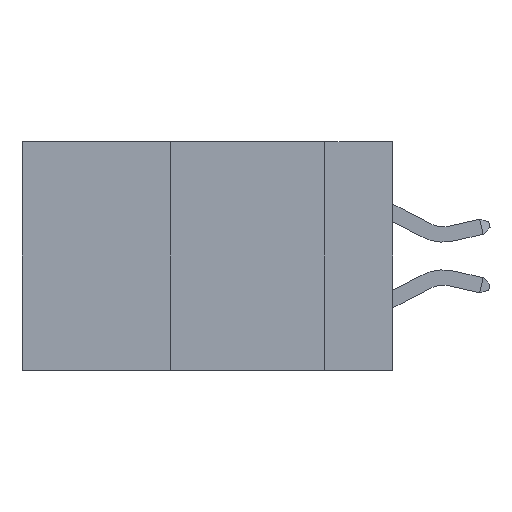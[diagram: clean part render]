
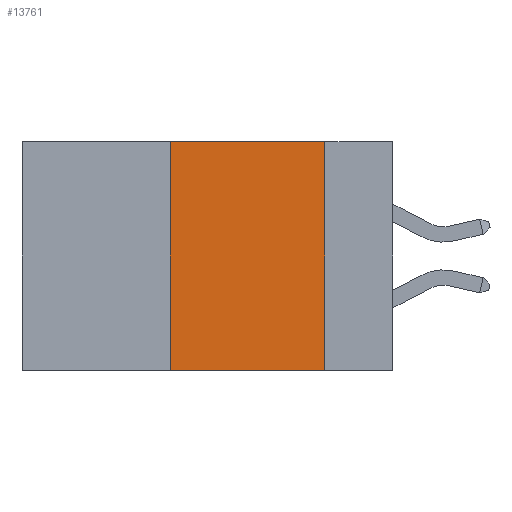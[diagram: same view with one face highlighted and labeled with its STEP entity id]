
A CAD part, left-side view. The second image highlights one B-rep face of the part: STEP entity #13761.
In plain terms, the highlighted planar face has unit normal (-1, 0, 0).
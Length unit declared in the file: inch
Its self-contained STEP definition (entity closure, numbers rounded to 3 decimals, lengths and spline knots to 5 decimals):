
#964 = DIRECTION ( 'NONE',  ( 1., 0., 0. ) ) ;
#1070 = VECTOR ( 'NONE', #2989, 39.37008 ) ;
#1494 = ORIENTED_EDGE ( 'NONE', *, *, #7366, .F. ) ;
#1691 = LINE ( 'NONE', #11585, #4032 ) ;
#1706 = CARTESIAN_POINT ( 'NONE',  ( 0., 0.36, 0. ) ) ;
#2989 = DIRECTION ( 'NONE',  ( 0., 0., 1. ) ) ;
#4032 = VECTOR ( 'NONE', #7355, 39.37008 ) ;
#4509 = ORIENTED_EDGE ( 'NONE', *, *, #10254, .T. ) ;
#5245 = CARTESIAN_POINT ( 'NONE',  ( 0., 0.11, -0.37 ) ) ;
#5344 = VERTEX_POINT ( 'NONE', #13307 ) ;
#5580 = CARTESIAN_POINT ( 'NONE',  ( 0., 0.36, 0. ) ) ;
#5608 = VECTOR ( 'NONE', #14240, 39.37008 ) ;
#6474 = ORIENTED_EDGE ( 'NONE', *, *, #16320, .F. ) ;
#7355 = DIRECTION ( 'NONE',  ( 0., -1., 0. ) ) ;
#7366 = EDGE_CURVE ( 'NONE', #11737, #9179, #15562, .T. ) ;
#7612 = AXIS2_PLACEMENT_3D ( 'NONE', #13719, #964, #9203 ) ;
#8470 = VECTOR ( 'NONE', #14599, 39.37008 ) ;
#9057 = LINE ( 'NONE', #12007, #8470 ) ;
#9179 = VERTEX_POINT ( 'NONE', #5580 ) ;
#9203 = DIRECTION ( 'NONE',  ( 0., 0., -1. ) ) ;
#9812 = CARTESIAN_POINT ( 'NONE',  ( 0., 0.36, -0.37 ) ) ;
#10254 = EDGE_CURVE ( 'NONE', #11737, #14271, #1691, .T. ) ;
#10599 = EDGE_LOOP ( 'NONE', ( #16565, #6474, #1494, #4509 ) ) ;
#11475 = LINE ( 'NONE', #12768, #5608 ) ;
#11585 = CARTESIAN_POINT ( 'NONE',  ( 0., 0.6, -0.37 ) ) ;
#11737 = VERTEX_POINT ( 'NONE', #9812 ) ;
#12007 = CARTESIAN_POINT ( 'NONE',  ( 0., 0.11, 0. ) ) ;
#12240 = PLANE ( 'NONE',  #7612 ) ;
#12704 = EDGE_CURVE ( 'NONE', #5344, #14271, #9057, .T. ) ;
#12768 = CARTESIAN_POINT ( 'NONE',  ( 0., 0.6, 0. ) ) ;
#13307 = CARTESIAN_POINT ( 'NONE',  ( 0., 0.11, 0. ) ) ;
#13719 = CARTESIAN_POINT ( 'NONE',  ( 0., 0.6, 0. ) ) ;
#13761 = ADVANCED_FACE ( 'NONE', ( #15107 ), #12240, .F. ) ;
#14240 = DIRECTION ( 'NONE',  ( 0., -1., 0. ) ) ;
#14271 = VERTEX_POINT ( 'NONE', #5245 ) ;
#14599 = DIRECTION ( 'NONE',  ( 0., 0., -1. ) ) ;
#15107 = FACE_OUTER_BOUND ( 'NONE', #10599, .T. ) ;
#15562 = LINE ( 'NONE', #1706, #1070 ) ;
#16320 = EDGE_CURVE ( 'NONE', #9179, #5344, #11475, .T. ) ;
#16565 = ORIENTED_EDGE ( 'NONE', *, *, #12704, .F. ) ;
